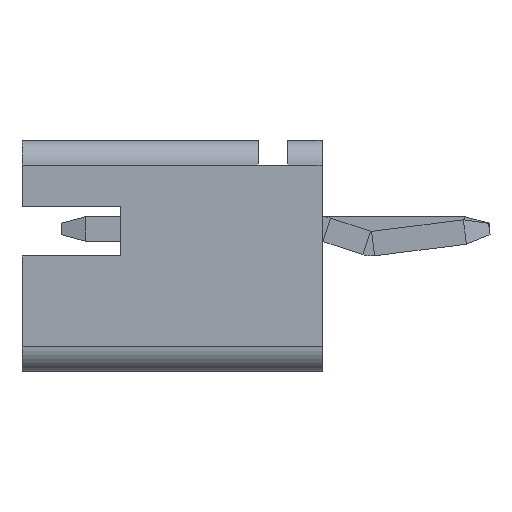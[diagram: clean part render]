
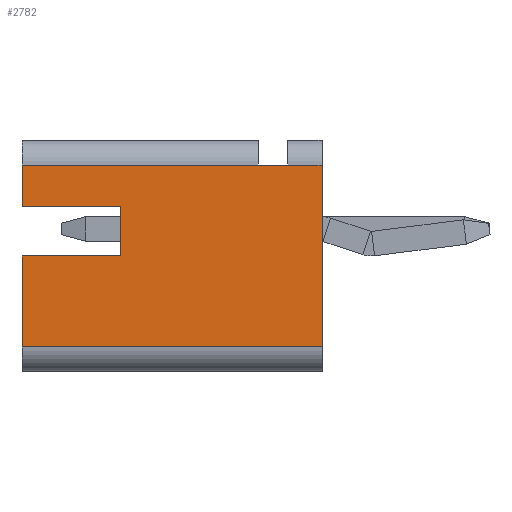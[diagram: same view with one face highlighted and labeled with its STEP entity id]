
A CAD part, left-side view. The second image highlights one B-rep face of the part: STEP entity #2782.
In plain terms, the highlighted planar face has unit normal (-1, 0, 0).
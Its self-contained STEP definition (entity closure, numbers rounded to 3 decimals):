
#7 = ORIENTED_EDGE ( 'NONE', *, *, #3827, .F. ) ;
#16 = ORIENTED_EDGE ( 'NONE', *, *, #1694, .T. ) ;
#63 = CARTESIAN_POINT ( 'NONE',  ( -2., 6.1, 0.45 ) ) ;
#181 = VERTEX_POINT ( 'NONE', #4420 ) ;
#281 = CARTESIAN_POINT ( 'NONE',  ( -2., 0., 1.3 ) ) ;
#338 = CARTESIAN_POINT ( 'NONE',  ( -2., 0., 0. ) ) ;
#409 = LINE ( 'NONE', #2666, #956 ) ;
#428 = LINE ( 'NONE', #2336, #1588 ) ;
#465 = DIRECTION ( 'NONE',  ( 0., -1., 0. ) ) ;
#585 = VECTOR ( 'NONE', #1689, 1000. ) ;
#591 = VECTOR ( 'NONE', #465, 1000. ) ;
#648 = VERTEX_POINT ( 'NONE', #2861 ) ;
#724 = DIRECTION ( 'NONE',  ( 0., 1., 0. ) ) ;
#901 = VECTOR ( 'NONE', #3380, 1000. ) ;
#928 = CARTESIAN_POINT ( 'NONE',  ( -2., 6.1, 1.8 ) ) ;
#956 = VECTOR ( 'NONE', #3021, 1000. ) ;
#1154 = CARTESIAN_POINT ( 'NONE',  ( -2., 6.1, -2.4 ) ) ;
#1187 = VECTOR ( 'NONE', #724, 1000. ) ;
#1194 = CARTESIAN_POINT ( 'NONE',  ( -2., 6.1, -0.55 ) ) ;
#1213 = ORIENTED_EDGE ( 'NONE', *, *, #2024, .F. ) ;
#1394 = VERTEX_POINT ( 'NONE', #2035 ) ;
#1471 = VECTOR ( 'NONE', #1518, 1000. ) ;
#1518 = DIRECTION ( 'NONE',  ( 0., 0., -1. ) ) ;
#1529 = ORIENTED_EDGE ( 'NONE', *, *, #2018, .F. ) ;
#1577 = VERTEX_POINT ( 'NONE', #3440 ) ;
#1588 = VECTOR ( 'NONE', #3079, 1000. ) ;
#1610 = ORIENTED_EDGE ( 'NONE', *, *, #2653, .F. ) ;
#1689 = DIRECTION ( 'NONE',  ( 0., -1., 0. ) ) ;
#1694 = EDGE_CURVE ( 'NONE', #3804, #2659, #428, .T. ) ;
#1700 = VERTEX_POINT ( 'NONE', #4470 ) ;
#1809 = ORIENTED_EDGE ( 'NONE', *, *, #3418, .F. ) ;
#1945 = CARTESIAN_POINT ( 'NONE',  ( -2., 0., 1.3 ) ) ;
#1950 = VERTEX_POINT ( 'NONE', #4019 ) ;
#2018 = EDGE_CURVE ( 'NONE', #3919, #2659, #2538, .T. ) ;
#2024 = EDGE_CURVE ( 'NONE', #181, #1700, #2147, .T. ) ;
#2035 = CARTESIAN_POINT ( 'NONE',  ( -2., 4.1, 0.45 ) ) ;
#2083 = LINE ( 'NONE', #3048, #585 ) ;
#2147 = LINE ( 'NONE', #2931, #591 ) ;
#2336 = CARTESIAN_POINT ( 'NONE',  ( -2., 0., -2.4 ) ) ;
#2436 = EDGE_CURVE ( 'NONE', #1394, #1577, #3145, .T. ) ;
#2521 = LINE ( 'NONE', #1945, #3573 ) ;
#2538 = LINE ( 'NONE', #2572, #1471 ) ;
#2572 = CARTESIAN_POINT ( 'NONE',  ( -2., 0., 1.8 ) ) ;
#2584 = VECTOR ( 'NONE', #3414, 1000. ) ;
#2616 = AXIS2_PLACEMENT_3D ( 'NONE', #338, #2768, #3892 ) ;
#2638 = LINE ( 'NONE', #928, #2584 ) ;
#2653 = EDGE_CURVE ( 'NONE', #1950, #2754, #2083, .T. ) ;
#2659 = VERTEX_POINT ( 'NONE', #4494 ) ;
#2666 = CARTESIAN_POINT ( 'NONE',  ( -2., 0., 1.3 ) ) ;
#2754 = VERTEX_POINT ( 'NONE', #2797 ) ;
#2768 = DIRECTION ( 'NONE',  ( 1., 0., 0. ) ) ;
#2782 = ADVANCED_FACE ( 'NONE', ( #3246 ), #3132, .F. ) ;
#2797 = CARTESIAN_POINT ( 'NONE',  ( -2., 0.7, 1.3 ) ) ;
#2861 = CARTESIAN_POINT ( 'NONE',  ( -2., 6.1, 1.3 ) ) ;
#2917 = LINE ( 'NONE', #1194, #4538 ) ;
#2931 = CARTESIAN_POINT ( 'NONE',  ( -2., 6.1, -0.55 ) ) ;
#2956 = EDGE_CURVE ( 'NONE', #3804, #181, #2917, .T. ) ;
#3021 = DIRECTION ( 'NONE',  ( 0., 1., 0. ) ) ;
#3048 = CARTESIAN_POINT ( 'NONE',  ( -2., 1.3, 1.3 ) ) ;
#3068 = CARTESIAN_POINT ( 'NONE',  ( -2., 4.1, 0.45 ) ) ;
#3079 = DIRECTION ( 'NONE',  ( 0., -1., 0. ) ) ;
#3132 = PLANE ( 'NONE',  #2616 ) ;
#3145 = LINE ( 'NONE', #63, #1187 ) ;
#3212 = EDGE_CURVE ( 'NONE', #1950, #648, #2521, .T. ) ;
#3246 = FACE_OUTER_BOUND ( 'NONE', #4482, .T. ) ;
#3269 = DIRECTION ( 'NONE',  ( 0., 0., 1. ) ) ;
#3380 = DIRECTION ( 'NONE',  ( 0., 0., 1. ) ) ;
#3414 = DIRECTION ( 'NONE',  ( 0., 0., 1. ) ) ;
#3418 = EDGE_CURVE ( 'NONE', #1577, #648, #2638, .T. ) ;
#3439 = EDGE_CURVE ( 'NONE', #3919, #2754, #409, .T. ) ;
#3440 = CARTESIAN_POINT ( 'NONE',  ( -2., 6.1, 0.45 ) ) ;
#3573 = VECTOR ( 'NONE', #3684, 1000. ) ;
#3684 = DIRECTION ( 'NONE',  ( 0., 1., 0. ) ) ;
#3706 = ORIENTED_EDGE ( 'NONE', *, *, #2436, .F. ) ;
#3804 = VERTEX_POINT ( 'NONE', #1154 ) ;
#3827 = EDGE_CURVE ( 'NONE', #1700, #1394, #4355, .T. ) ;
#3892 = DIRECTION ( 'NONE',  ( 0., 0., -1. ) ) ;
#3919 = VERTEX_POINT ( 'NONE', #281 ) ;
#4019 = CARTESIAN_POINT ( 'NONE',  ( -2., 1.3, 1.3 ) ) ;
#4040 = ORIENTED_EDGE ( 'NONE', *, *, #3439, .T. ) ;
#4355 = LINE ( 'NONE', #3068, #901 ) ;
#4420 = CARTESIAN_POINT ( 'NONE',  ( -2., 6.1, -0.55 ) ) ;
#4421 = ORIENTED_EDGE ( 'NONE', *, *, #2956, .F. ) ;
#4470 = CARTESIAN_POINT ( 'NONE',  ( -2., 4.1, -0.55 ) ) ;
#4482 = EDGE_LOOP ( 'NONE', ( #4421, #16, #1529, #4040, #1610, #4536, #1809, #3706, #7, #1213 ) ) ;
#4494 = CARTESIAN_POINT ( 'NONE',  ( -2., 0., -2.4 ) ) ;
#4536 = ORIENTED_EDGE ( 'NONE', *, *, #3212, .T. ) ;
#4538 = VECTOR ( 'NONE', #3269, 1000. ) ;
